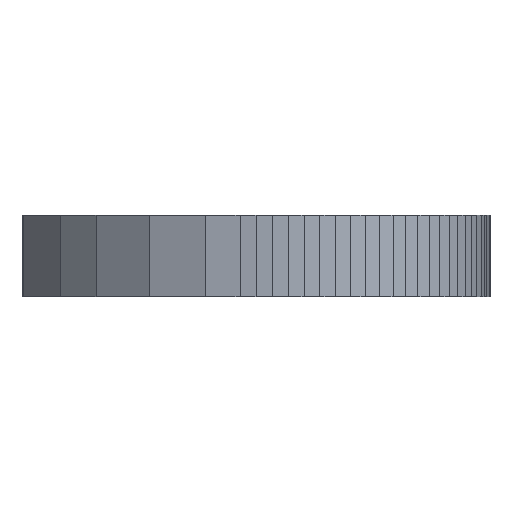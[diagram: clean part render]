
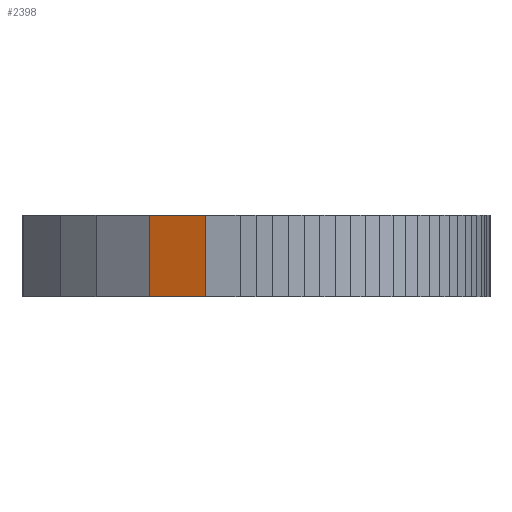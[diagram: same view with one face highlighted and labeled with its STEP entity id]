
A CAD part, left-side view. The second image highlights one B-rep face of the part: STEP entity #2398.
In plain terms, the highlighted planar face has unit normal (-0.933, 0.359, 0).
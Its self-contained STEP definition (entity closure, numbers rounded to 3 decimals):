
#2342=CARTESIAN_POINT('',(-34.478,5.025,0.0));
#2343=VERTEX_POINT('',#2342);
#2351=CARTESIAN_POINT('',(-34.478,5.025,11.0));
#2352=VERTEX_POINT('',#2351);
#2359=CARTESIAN_POINT('',(-34.478,5.025,0.0));
#2360=DIRECTION('',(0.0,0.0,1.0));
#2361=VECTOR('',#2360,11.0);
#2362=LINE('',#2359,#2361);
#2363=EDGE_CURVE('',#2343,#2352,#2362,.T.);
#2368=CARTESIAN_POINT('',(-31.571,12.584,0.0));
#2369=DIRECTION('',(-0.933,0.359,0.0));
#2370=DIRECTION('',(-0.359,-0.933,0.0));
#2371=AXIS2_PLACEMENT_3D('',#2368,#2369,#2370);
#2372=PLANE('',#2371);
#2373=CARTESIAN_POINT('',(-31.571,12.584,0.0));
#2374=VERTEX_POINT('',#2373);
#2375=CARTESIAN_POINT('',(-31.571,12.584,0.0));
#2376=DIRECTION('',(-0.359,-0.933,0.0));
#2377=VECTOR('',#2376,8.098);
#2378=LINE('',#2375,#2377);
#2379=EDGE_CURVE('',#2374,#2343,#2378,.T.);
#2380=ORIENTED_EDGE('',*,*,#2379,.T.);
#2381=ORIENTED_EDGE('',*,*,#2363,.T.);
#2382=CARTESIAN_POINT('',(-31.571,12.584,11.0));
#2383=VERTEX_POINT('',#2382);
#2384=CARTESIAN_POINT('',(-31.571,12.584,11.0));
#2385=DIRECTION('',(-0.359,-0.933,0.0));
#2386=VECTOR('',#2385,8.098);
#2387=LINE('',#2384,#2386);
#2388=EDGE_CURVE('',#2383,#2352,#2387,.T.);
#2389=ORIENTED_EDGE('',*,*,#2388,.F.);
#2390=CARTESIAN_POINT('',(-31.571,12.584,0.0));
#2391=DIRECTION('',(0.0,0.0,1.0));
#2392=VECTOR('',#2391,11.0);
#2393=LINE('',#2390,#2392);
#2394=EDGE_CURVE('',#2374,#2383,#2393,.T.);
#2395=ORIENTED_EDGE('',*,*,#2394,.F.);
#2396=EDGE_LOOP('',(#2380,#2381,#2389,#2395));
#2397=FACE_OUTER_BOUND('',#2396,.T.);
#2398=ADVANCED_FACE('',(#2397),#2372,.T.);
